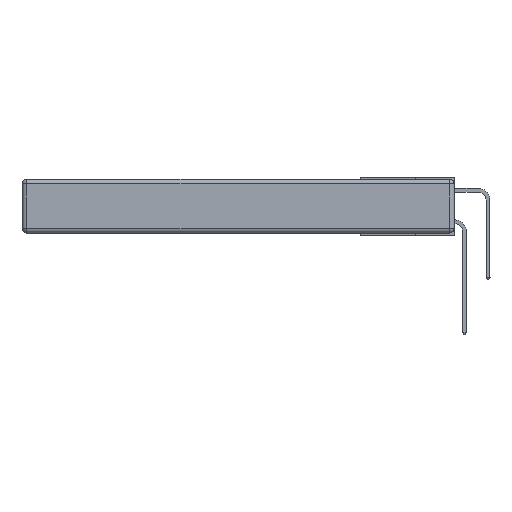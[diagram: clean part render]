
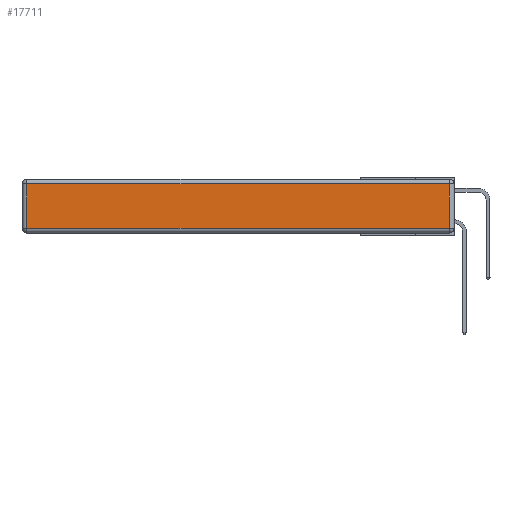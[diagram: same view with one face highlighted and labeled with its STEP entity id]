
A CAD part, left-side view. The second image highlights one B-rep face of the part: STEP entity #17711.
In plain terms, the highlighted planar face has unit normal (-1, 0, 0).
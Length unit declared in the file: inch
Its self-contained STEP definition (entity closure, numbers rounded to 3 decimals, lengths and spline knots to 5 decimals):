
#49 = DIRECTION ( 'NONE',  ( 0., -1., 0. ) ) ;
#320 = CARTESIAN_POINT ( 'NONE',  ( 0., 0.03, -0.313 ) ) ;
#812 = CARTESIAN_POINT ( 'NONE',  ( 0., 0.03, -0.343 ) ) ;
#905 = VERTEX_POINT ( 'NONE', #4339 ) ;
#1169 = DIRECTION ( 'NONE',  ( 0., 0., 1. ) ) ;
#1379 = VECTOR ( 'NONE', #11165, 39.37008 ) ;
#1386 = AXIS2_PLACEMENT_3D ( 'NONE', #7976, #21190, #1169 ) ;
#1425 = CARTESIAN_POINT ( 'NONE',  ( 0., 0.03, -0.03 ) ) ;
#1598 = VERTEX_POINT ( 'NONE', #6218 ) ;
#1742 = LINE ( 'NONE', #4772, #20269 ) ;
#3739 = ORIENTED_EDGE ( 'NONE', *, *, #12691, .T. ) ;
#4304 = LINE ( 'NONE', #14604, #5324 ) ;
#4339 = CARTESIAN_POINT ( 'NONE',  ( 0., 2.72, -0.313 ) ) ;
#4772 = CARTESIAN_POINT ( 'NONE',  ( 0., 0., -0.313 ) ) ;
#5044 = EDGE_CURVE ( 'NONE', #905, #11261, #1742, .T. ) ;
#5324 = VECTOR ( 'NONE', #14734, 39.37008 ) ;
#6092 = DIRECTION ( 'NONE',  ( 0., 0., -1. ) ) ;
#6218 = CARTESIAN_POINT ( 'NONE',  ( 0., 2.72, -0.03 ) ) ;
#7184 = EDGE_CURVE ( 'NONE', #11261, #13454, #8950, .T. ) ;
#7976 = CARTESIAN_POINT ( 'NONE',  ( 0., 0., -0.343 ) ) ;
#8270 = PLANE ( 'NONE',  #1386 ) ;
#8950 = LINE ( 'NONE', #812, #1379 ) ;
#10522 = EDGE_CURVE ( 'NONE', #13454, #1598, #4304, .T. ) ;
#11165 = DIRECTION ( 'NONE',  ( 0., 0., 1. ) ) ;
#11261 = VERTEX_POINT ( 'NONE', #320 ) ;
#11841 = VECTOR ( 'NONE', #6092, 39.37008 ) ;
#11923 = FACE_OUTER_BOUND ( 'NONE', #20719, .T. ) ;
#12691 = EDGE_CURVE ( 'NONE', #1598, #905, #20147, .T. ) ;
#13454 = VERTEX_POINT ( 'NONE', #1425 ) ;
#14530 = ORIENTED_EDGE ( 'NONE', *, *, #7184, .T. ) ;
#14604 = CARTESIAN_POINT ( 'NONE',  ( 0., 2.75, -0.03 ) ) ;
#14734 = DIRECTION ( 'NONE',  ( 0., 1., 0. ) ) ;
#16204 = CARTESIAN_POINT ( 'NONE',  ( 0., 2.72, -0.343 ) ) ;
#17276 = ORIENTED_EDGE ( 'NONE', *, *, #5044, .T. ) ;
#17711 = ADVANCED_FACE ( 'NONE', ( #11923 ), #8270, .T. ) ;
#20147 = LINE ( 'NONE', #16204, #11841 ) ;
#20269 = VECTOR ( 'NONE', #49, 39.37008 ) ;
#20482 = ORIENTED_EDGE ( 'NONE', *, *, #10522, .T. ) ;
#20719 = EDGE_LOOP ( 'NONE', ( #17276, #14530, #20482, #3739 ) ) ;
#21190 = DIRECTION ( 'NONE',  ( -1., 0., 0. ) ) ;
